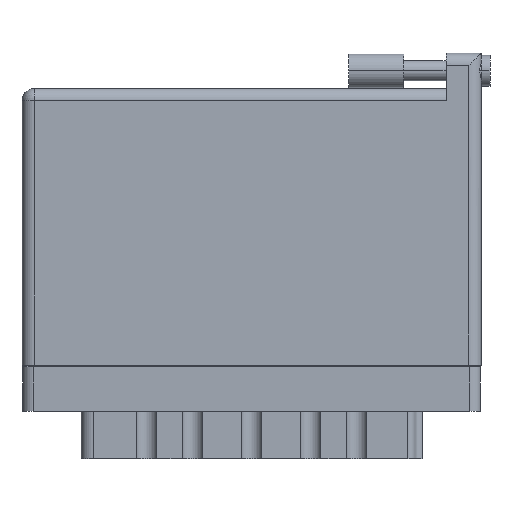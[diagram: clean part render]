
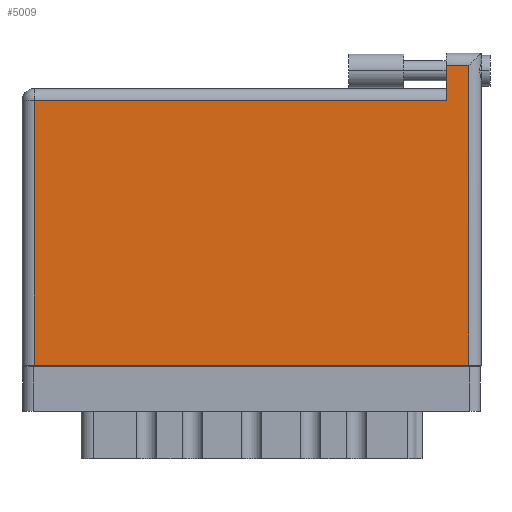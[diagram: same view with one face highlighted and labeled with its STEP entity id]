
A CAD part, front view. The second image highlights one B-rep face of the part: STEP entity #5009.
In plain terms, the highlighted face is planar.
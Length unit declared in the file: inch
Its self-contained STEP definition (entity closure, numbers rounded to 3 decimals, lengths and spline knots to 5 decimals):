
#1135 = CARTESIAN_POINT ( 'NONE',  ( 2.403, 1.496, 0. ) ) ;
#2032 = CARTESIAN_POINT ( 'NONE',  ( 0.07, 0., 0. ) ) ;
#2455 = PLANE ( 'NONE',  #18459 ) ;
#3296 = DIRECTION ( 'NONE',  ( -1., 0., 0. ) ) ;
#5009 = ADVANCED_FACE ( 'NONE', ( #7604 ), #2455, .F. ) ;
#5076 = VECTOR ( 'NONE', #32263, 39.37008 ) ;
#6166 = LINE ( 'NONE', #39031, #5076 ) ;
#6960 = DIRECTION ( 'NONE',  ( -1., 0., 0. ) ) ;
#7604 = FACE_OUTER_BOUND ( 'NONE', #13621, .T. ) ;
#7916 = VECTOR ( 'NONE', #37026, 39.37008 ) ;
#8154 = CARTESIAN_POINT ( 'NONE',  ( 2.53, 1.696, 0. ) ) ;
#8158 = CARTESIAN_POINT ( 'NONE',  ( 2.53, 1.766, 0. ) ) ;
#8851 = EDGE_CURVE ( 'NONE', #25177, #20211, #41766, .T. ) ;
#8934 = LINE ( 'NONE', #14093, #35457 ) ;
#9484 = CARTESIAN_POINT ( 'NONE',  ( 0., 1.566, 0. ) ) ;
#10581 = CARTESIAN_POINT ( 'NONE',  ( 0., 1.696, 0. ) ) ;
#12368 = CARTESIAN_POINT ( 'NONE',  ( 0.07, 0., 0. ) ) ;
#13112 = CARTESIAN_POINT ( 'NONE',  ( 0.07, 1.496, 0. ) ) ;
#13621 = EDGE_LOOP ( 'NONE', ( #32088, #15329, #21068, #37869, #41973, #35525 ) ) ;
#14093 = CARTESIAN_POINT ( 'NONE',  ( 0., 0., 0. ) ) ;
#15092 = VERTEX_POINT ( 'NONE', #1135 ) ;
#15231 = DIRECTION ( 'NONE',  ( 0., 1., 0. ) ) ;
#15329 = ORIENTED_EDGE ( 'NONE', *, *, #37960, .T. ) ;
#17170 = LINE ( 'NONE', #40861, #22578 ) ;
#18459 = AXIS2_PLACEMENT_3D ( 'NONE', #9484, #37603, #41069 ) ;
#20211 = VERTEX_POINT ( 'NONE', #37642 ) ;
#21068 = ORIENTED_EDGE ( 'NONE', *, *, #8851, .T. ) ;
#21416 = EDGE_CURVE ( 'NONE', #15092, #37366, #17170, .T. ) ;
#21642 = EDGE_CURVE ( 'NONE', #37366, #29189, #41482, .T. ) ;
#22578 = VECTOR ( 'NONE', #6960, 39.37008 ) ;
#25177 = VERTEX_POINT ( 'NONE', #8154 ) ;
#29189 = VERTEX_POINT ( 'NONE', #12368 ) ;
#29348 = VECTOR ( 'NONE', #3296, 39.37008 ) ;
#29735 = LINE ( 'NONE', #8158, #31345 ) ;
#31345 = VECTOR ( 'NONE', #15231, 39.37008 ) ;
#32088 = ORIENTED_EDGE ( 'NONE', *, *, #35116, .T. ) ;
#32263 = DIRECTION ( 'NONE',  ( 0., -1., 0. ) ) ;
#35008 = CARTESIAN_POINT ( 'NONE',  ( 2.53, 0., 0. ) ) ;
#35116 = EDGE_CURVE ( 'NONE', #29189, #38916, #8934, .T. ) ;
#35457 = VECTOR ( 'NONE', #38469, 39.37008 ) ;
#35505 = EDGE_CURVE ( 'NONE', #20211, #15092, #6166, .T. ) ;
#35525 = ORIENTED_EDGE ( 'NONE', *, *, #21642, .T. ) ;
#37026 = DIRECTION ( 'NONE',  ( 0., -1., 0. ) ) ;
#37366 = VERTEX_POINT ( 'NONE', #13112 ) ;
#37603 = DIRECTION ( 'NONE',  ( 0., 0., -1. ) ) ;
#37642 = CARTESIAN_POINT ( 'NONE',  ( 2.403, 1.696, 0. ) ) ;
#37869 = ORIENTED_EDGE ( 'NONE', *, *, #35505, .T. ) ;
#37960 = EDGE_CURVE ( 'NONE', #38916, #25177, #29735, .T. ) ;
#38469 = DIRECTION ( 'NONE',  ( 1., 0., 0. ) ) ;
#38916 = VERTEX_POINT ( 'NONE', #35008 ) ;
#39031 = CARTESIAN_POINT ( 'NONE',  ( 2.403, 1.766, 0. ) ) ;
#40861 = CARTESIAN_POINT ( 'NONE',  ( 0., 1.496, 0. ) ) ;
#41069 = DIRECTION ( 'NONE',  ( -1., 0., 0. ) ) ;
#41482 = LINE ( 'NONE', #2032, #7916 ) ;
#41766 = LINE ( 'NONE', #10581, #29348 ) ;
#41973 = ORIENTED_EDGE ( 'NONE', *, *, #21416, .T. ) ;
